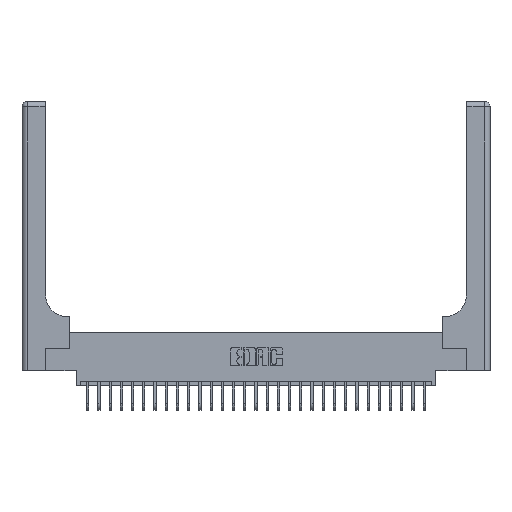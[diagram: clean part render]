
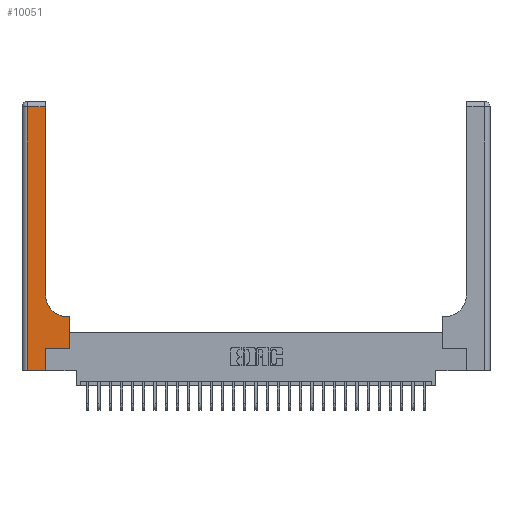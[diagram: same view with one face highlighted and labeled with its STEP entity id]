
A CAD part, top view. The second image highlights one B-rep face of the part: STEP entity #10051.
In plain terms, the highlighted planar face has unit normal (0, 0, 1).
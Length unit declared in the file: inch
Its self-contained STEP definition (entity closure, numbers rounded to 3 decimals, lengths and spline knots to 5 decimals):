
#350 = VECTOR ( 'NONE', #1828, 39.37008 ) ;
#510 = LINE ( 'NONE', #946, #14562 ) ;
#579 = VERTEX_POINT ( 'NONE', #7284 ) ;
#946 = CARTESIAN_POINT ( 'NONE',  ( 0.26, 0.6, 0.37 ) ) ;
#984 = CARTESIAN_POINT ( 'NONE',  ( 0.265, 0.25, 0.37 ) ) ;
#1563 = VERTEX_POINT ( 'NONE', #984 ) ;
#1691 = EDGE_CURVE ( 'NONE', #579, #23989, #4239, .T. ) ;
#1828 = DIRECTION ( 'NONE',  ( 0., 1., 0. ) ) ;
#2047 = CARTESIAN_POINT ( 'NONE',  ( 0.26, 0.85, 0.37 ) ) ;
#2455 = CARTESIAN_POINT ( 'NONE',  ( 0.51, 0.85, 0.37 ) ) ;
#2652 = CARTESIAN_POINT ( 'NONE',  ( 0.06, 2.94, 0.37 ) ) ;
#2656 = DIRECTION ( 'NONE',  ( 0., 0., -1. ) ) ;
#3890 = VERTEX_POINT ( 'NONE', #15102 ) ;
#3948 = DIRECTION ( 'NONE',  ( -1., 0., 0. ) ) ;
#4152 = AXIS2_PLACEMENT_3D ( 'NONE', #22951, #2656, #3948 ) ;
#4239 = LINE ( 'NONE', #26466, #17883 ) ;
#5895 = EDGE_CURVE ( 'NONE', #23302, #3890, #13080, .T. ) ;
#6075 = LINE ( 'NONE', #12035, #17821 ) ;
#6624 = DIRECTION ( 'NONE',  ( 1., 0., 0. ) ) ;
#6796 = AXIS2_PLACEMENT_3D ( 'NONE', #2455, #11344, #7188 ) ;
#7188 = DIRECTION ( 'NONE',  ( 1., 0., 0. ) ) ;
#7284 = CARTESIAN_POINT ( 'NONE',  ( 0.528, 0.25, 0.37 ) ) ;
#8005 = VERTEX_POINT ( 'NONE', #22738 ) ;
#8637 = EDGE_CURVE ( 'NONE', #14776, #9242, #6075, .T. ) ;
#9242 = VERTEX_POINT ( 'NONE', #27057 ) ;
#9569 = ORIENTED_EDGE ( 'NONE', *, *, #1691, .T. ) ;
#10051 = ADVANCED_FACE ( 'NONE', ( #18359 ), #27401, .F. ) ;
#10520 = EDGE_CURVE ( 'NONE', #23989, #8005, #510, .T. ) ;
#10721 = EDGE_CURVE ( 'NONE', #1563, #579, #22956, .T. ) ;
#10911 = DIRECTION ( 'NONE',  ( 0., 1., 0. ) ) ;
#11151 = CARTESIAN_POINT ( 'NONE',  ( 0.265, 0., 0.37 ) ) ;
#11344 = DIRECTION ( 'NONE',  ( 0., 0., -1. ) ) ;
#11415 = ORIENTED_EDGE ( 'NONE', *, *, #5895, .T. ) ;
#12035 = CARTESIAN_POINT ( 'NONE',  ( 0.06, 3., 0.37 ) ) ;
#13080 = LINE ( 'NONE', #26719, #350 ) ;
#13555 = ORIENTED_EDGE ( 'NONE', *, *, #13786, .T. ) ;
#13786 = EDGE_CURVE ( 'NONE', #3890, #14776, #16887, .T. ) ;
#14111 = VERTEX_POINT ( 'NONE', #11151 ) ;
#14562 = VECTOR ( 'NONE', #18572, 39.37008 ) ;
#14776 = VERTEX_POINT ( 'NONE', #2652 ) ;
#15102 = CARTESIAN_POINT ( 'NONE',  ( 0.26, 2.94, 0.37 ) ) ;
#16382 = VECTOR ( 'NONE', #6624, 39.37008 ) ;
#16627 = DIRECTION ( 'NONE',  ( 0., -1., 0. ) ) ;
#16887 = LINE ( 'NONE', #24001, #22259 ) ;
#17821 = VECTOR ( 'NONE', #16627, 39.37008 ) ;
#17883 = VECTOR ( 'NONE', #10911, 39.37008 ) ;
#18359 = FACE_OUTER_BOUND ( 'NONE', #18900, .T. ) ;
#18572 = DIRECTION ( 'NONE',  ( -1., 0., 0. ) ) ;
#18900 = EDGE_LOOP ( 'NONE', ( #11415, #13555, #29145, #26484, #22469, #19842, #9569, #25028, #23238 ) ) ;
#19009 = EDGE_CURVE ( 'NONE', #8005, #23302, #25241, .T. ) ;
#19409 = DIRECTION ( 'NONE',  ( -1., 0., 0. ) ) ;
#19842 = ORIENTED_EDGE ( 'NONE', *, *, #10721, .T. ) ;
#19961 = CARTESIAN_POINT ( 'NONE',  ( 0., 0., 0.37 ) ) ;
#20249 = LINE ( 'NONE', #19961, #16382 ) ;
#20271 = VECTOR ( 'NONE', #24875, 39.37008 ) ;
#20579 = CARTESIAN_POINT ( 'NONE',  ( 0.265, 0.25, 0.37 ) ) ;
#21512 = EDGE_CURVE ( 'NONE', #9242, #14111, #20249, .T. ) ;
#21541 = LINE ( 'NONE', #28371, #24621 ) ;
#22259 = VECTOR ( 'NONE', #19409, 39.37008 ) ;
#22469 = ORIENTED_EDGE ( 'NONE', *, *, #28379, .T. ) ;
#22738 = CARTESIAN_POINT ( 'NONE',  ( 0.51, 0.6, 0.37 ) ) ;
#22951 = CARTESIAN_POINT ( 'NONE',  ( 0., 3., 0.37 ) ) ;
#22956 = LINE ( 'NONE', #20579, #20271 ) ;
#23238 = ORIENTED_EDGE ( 'NONE', *, *, #19009, .T. ) ;
#23302 = VERTEX_POINT ( 'NONE', #2047 ) ;
#23422 = CARTESIAN_POINT ( 'NONE',  ( 0.528, 0.6, 0.37 ) ) ;
#23620 = DIRECTION ( 'NONE',  ( 0., 1., 0. ) ) ;
#23989 = VERTEX_POINT ( 'NONE', #23422 ) ;
#24001 = CARTESIAN_POINT ( 'NONE',  ( 0., 2.94, 0.37 ) ) ;
#24621 = VECTOR ( 'NONE', #23620, 39.37008 ) ;
#24875 = DIRECTION ( 'NONE',  ( 1., 0., 0. ) ) ;
#25028 = ORIENTED_EDGE ( 'NONE', *, *, #10520, .T. ) ;
#25241 = CIRCLE ( 'NONE', #6796, 0.25 ) ;
#26466 = CARTESIAN_POINT ( 'NONE',  ( 0.528, 0.25, 0.37 ) ) ;
#26484 = ORIENTED_EDGE ( 'NONE', *, *, #21512, .T. ) ;
#26719 = CARTESIAN_POINT ( 'NONE',  ( 0.26, 3., 0.37 ) ) ;
#27057 = CARTESIAN_POINT ( 'NONE',  ( 0.06, 0., 0.37 ) ) ;
#27401 = PLANE ( 'NONE',  #4152 ) ;
#28371 = CARTESIAN_POINT ( 'NONE',  ( 0.265, 0., 0.37 ) ) ;
#28379 = EDGE_CURVE ( 'NONE', #14111, #1563, #21541, .T. ) ;
#29145 = ORIENTED_EDGE ( 'NONE', *, *, #8637, .T. ) ;
